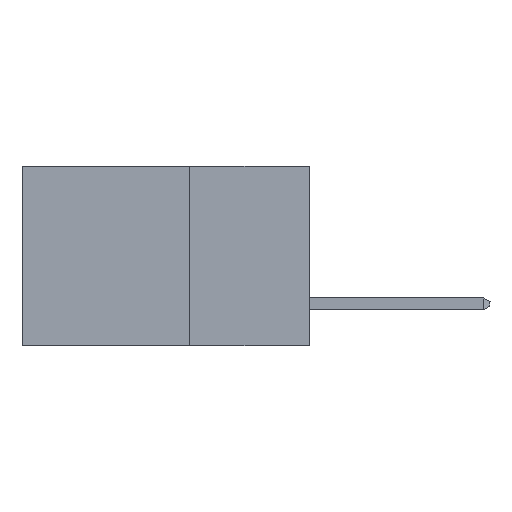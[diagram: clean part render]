
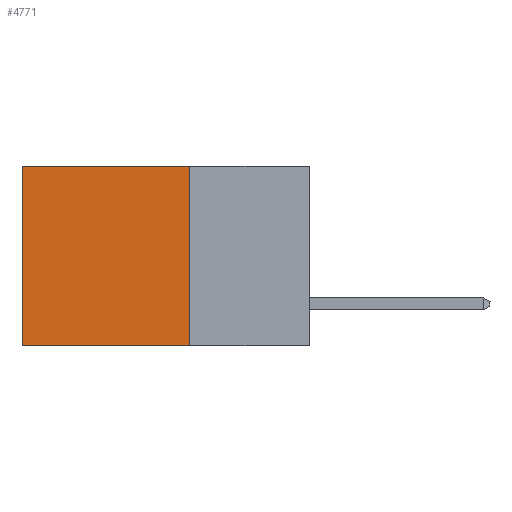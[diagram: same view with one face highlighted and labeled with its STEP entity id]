
A CAD part, left-side view. The second image highlights one B-rep face of the part: STEP entity #4771.
In plain terms, the highlighted planar face has unit normal (-1, 0, 0).
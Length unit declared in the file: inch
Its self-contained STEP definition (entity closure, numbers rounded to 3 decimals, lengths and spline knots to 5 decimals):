
#87 = PLANE ( 'NONE',  #698 ) ;
#543 = DIRECTION ( 'NONE',  ( 0., 1., 0. ) ) ;
#698 = AXIS2_PLACEMENT_3D ( 'NONE', #6147, #3152, #10962 ) ;
#929 = ORIENTED_EDGE ( 'NONE', *, *, #3835, .F. ) ;
#1145 = LINE ( 'NONE', #7463, #10771 ) ;
#1282 = VERTEX_POINT ( 'NONE', #10909 ) ;
#1337 = DIRECTION ( 'NONE',  ( 0., 1., 0. ) ) ;
#1423 = DIRECTION ( 'NONE',  ( 0., 0., -1. ) ) ;
#1593 = VERTEX_POINT ( 'NONE', #1734 ) ;
#1651 = ORIENTED_EDGE ( 'NONE', *, *, #6578, .T. ) ;
#1734 = CARTESIAN_POINT ( 'NONE',  ( 0.2875, 0.6, -0.375 ) ) ;
#1786 = CARTESIAN_POINT ( 'NONE',  ( 0.2875, 0.25, -0.375 ) ) ;
#2095 = FACE_OUTER_BOUND ( 'NONE', #3276, .T. ) ;
#2434 = CARTESIAN_POINT ( 'NONE',  ( 0.2875, 0.25, -0.375 ) ) ;
#2710 = EDGE_CURVE ( 'NONE', #1282, #1593, #12354, .T. ) ;
#3152 = DIRECTION ( 'NONE',  ( 1., 0., 0. ) ) ;
#3276 = EDGE_LOOP ( 'NONE', ( #5455, #929, #10297, #1651 ) ) ;
#3431 = LINE ( 'NONE', #2434, #7873 ) ;
#3488 = VECTOR ( 'NONE', #543, 39.37008 ) ;
#3835 = EDGE_CURVE ( 'NONE', #7947, #1593, #8795, .T. ) ;
#4666 = CARTESIAN_POINT ( 'NONE',  ( 0.2875, 0.25, -0.375 ) ) ;
#4771 = ADVANCED_FACE ( 'NONE', ( #2095 ), #87, .F. ) ;
#5210 = CARTESIAN_POINT ( 'NONE',  ( 0.2875, 0.6, -0.375 ) ) ;
#5455 = ORIENTED_EDGE ( 'NONE', *, *, #2710, .T. ) ;
#6147 = CARTESIAN_POINT ( 'NONE',  ( 0.2875, 0.25, -0.375 ) ) ;
#6355 = EDGE_CURVE ( 'NONE', #8886, #7947, #3431, .T. ) ;
#6578 = EDGE_CURVE ( 'NONE', #8886, #1282, #1145, .T. ) ;
#7463 = CARTESIAN_POINT ( 'NONE',  ( 0.2875, 0.25, 0. ) ) ;
#7873 = VECTOR ( 'NONE', #1423, 39.37008 ) ;
#7947 = VERTEX_POINT ( 'NONE', #1786 ) ;
#8795 = LINE ( 'NONE', #4666, #3488 ) ;
#8886 = VERTEX_POINT ( 'NONE', #9330 ) ;
#9330 = CARTESIAN_POINT ( 'NONE',  ( 0.2875, 0.25, 0. ) ) ;
#10297 = ORIENTED_EDGE ( 'NONE', *, *, #6355, .F. ) ;
#10415 = DIRECTION ( 'NONE',  ( 0., 0., -1. ) ) ;
#10771 = VECTOR ( 'NONE', #1337, 39.37008 ) ;
#10893 = VECTOR ( 'NONE', #10415, 39.37008 ) ;
#10909 = CARTESIAN_POINT ( 'NONE',  ( 0.2875, 0.6, 0. ) ) ;
#10962 = DIRECTION ( 'NONE',  ( 0., 0., -1. ) ) ;
#12354 = LINE ( 'NONE', #5210, #10893 ) ;
